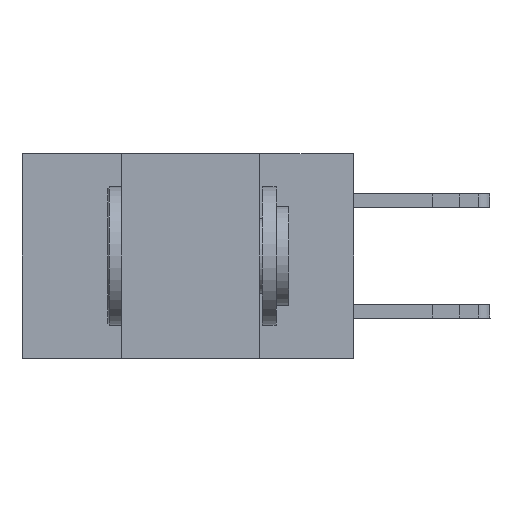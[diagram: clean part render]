
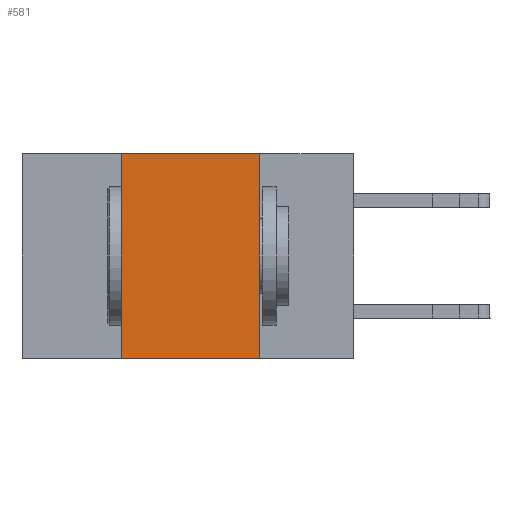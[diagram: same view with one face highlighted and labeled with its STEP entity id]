
A CAD part, left-side view. The second image highlights one B-rep face of the part: STEP entity #581.
In plain terms, the highlighted planar face has unit normal (-1, 0, 0).
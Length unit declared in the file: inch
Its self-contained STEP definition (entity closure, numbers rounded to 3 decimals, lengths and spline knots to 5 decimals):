
#110 = AXIS2_PLACEMENT_3D ( 'NONE', #17131, #10165, #17226 ) ;
#581 = ADVANCED_FACE ( 'NONE', ( #20374 ), #7498, .F. ) ;
#836 = CARTESIAN_POINT ( 'NONE',  ( 0., 0.42, 0. ) ) ;
#1940 = VECTOR ( 'NONE', #12241, 39.37008 ) ;
#3235 = VECTOR ( 'NONE', #18951, 39.37008 ) ;
#3651 = VECTOR ( 'NONE', #6871, 39.37008 ) ;
#4064 = VECTOR ( 'NONE', #4333, 39.37008 ) ;
#4323 = VERTEX_POINT ( 'NONE', #20004 ) ;
#4333 = DIRECTION ( 'NONE',  ( 0., 0., -1. ) ) ;
#5356 = VERTEX_POINT ( 'NONE', #15946 ) ;
#5748 = LINE ( 'NONE', #20078, #1940 ) ;
#5749 = EDGE_CURVE ( 'NONE', #14178, #4323, #14060, .T. ) ;
#6052 = VERTEX_POINT ( 'NONE', #836 ) ;
#6871 = DIRECTION ( 'NONE',  ( 0., 0., 1. ) ) ;
#7482 = CARTESIAN_POINT ( 'NONE',  ( 0., 0.17, 0. ) ) ;
#7498 = PLANE ( 'NONE',  #110 ) ;
#9298 = CARTESIAN_POINT ( 'NONE',  ( 0., 0.42, 0. ) ) ;
#9313 = EDGE_CURVE ( 'NONE', #14178, #6052, #14336, .T. ) ;
#9479 = ORIENTED_EDGE ( 'NONE', *, *, #9313, .F. ) ;
#10044 = EDGE_LOOP ( 'NONE', ( #18568, #11397, #9479, #19702 ) ) ;
#10165 = DIRECTION ( 'NONE',  ( 1., 0., 0. ) ) ;
#11292 = EDGE_CURVE ( 'NONE', #5356, #4323, #13794, .T. ) ;
#11397 = ORIENTED_EDGE ( 'NONE', *, *, #12398, .F. ) ;
#12241 = DIRECTION ( 'NONE',  ( 0., -1., 0. ) ) ;
#12398 = EDGE_CURVE ( 'NONE', #6052, #5356, #5748, .T. ) ;
#12797 = CARTESIAN_POINT ( 'NONE',  ( 0., 0.6, -0.37 ) ) ;
#13690 = CARTESIAN_POINT ( 'NONE',  ( 0., 0.42, -0.37 ) ) ;
#13794 = LINE ( 'NONE', #7482, #4064 ) ;
#14060 = LINE ( 'NONE', #12797, #3235 ) ;
#14178 = VERTEX_POINT ( 'NONE', #13690 ) ;
#14336 = LINE ( 'NONE', #9298, #3651 ) ;
#15946 = CARTESIAN_POINT ( 'NONE',  ( 0., 0.17, 0. ) ) ;
#17131 = CARTESIAN_POINT ( 'NONE',  ( 0., 0.6, 0. ) ) ;
#17226 = DIRECTION ( 'NONE',  ( 0., 0., -1. ) ) ;
#18568 = ORIENTED_EDGE ( 'NONE', *, *, #11292, .F. ) ;
#18951 = DIRECTION ( 'NONE',  ( 0., -1., 0. ) ) ;
#19702 = ORIENTED_EDGE ( 'NONE', *, *, #5749, .T. ) ;
#20004 = CARTESIAN_POINT ( 'NONE',  ( 0., 0.17, -0.37 ) ) ;
#20078 = CARTESIAN_POINT ( 'NONE',  ( 0., 0.6, 0. ) ) ;
#20374 = FACE_OUTER_BOUND ( 'NONE', #10044, .T. ) ;
